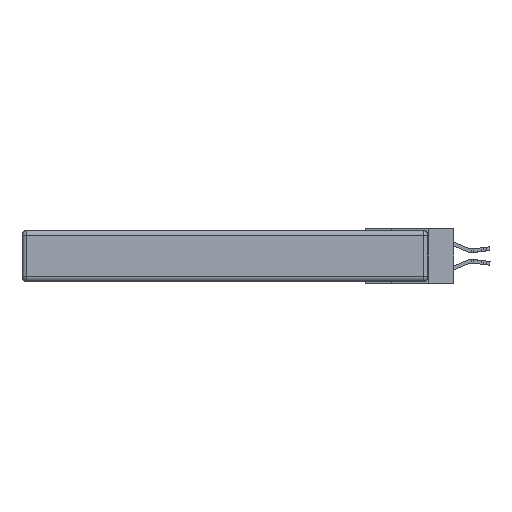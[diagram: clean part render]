
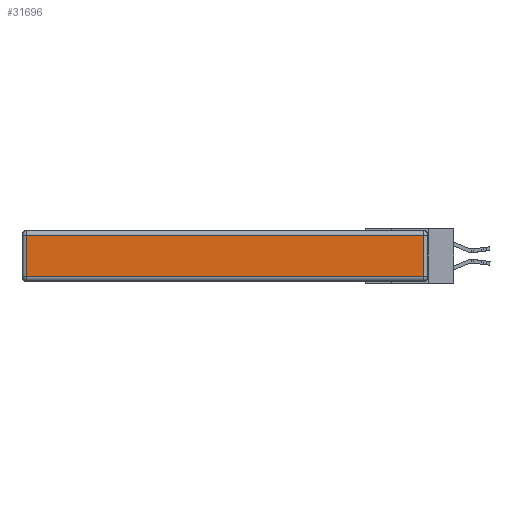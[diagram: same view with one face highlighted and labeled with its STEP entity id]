
A CAD part, left-side view. The second image highlights one B-rep face of the part: STEP entity #31696.
In plain terms, the highlighted planar face has unit normal (-1, 0, 0).
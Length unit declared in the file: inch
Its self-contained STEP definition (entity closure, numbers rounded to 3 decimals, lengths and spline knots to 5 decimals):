
#402 = DIRECTION ( 'NONE',  ( 0., 0., 1. ) ) ;
#422 = EDGE_LOOP ( 'NONE', ( #14379, #6504, #4582, #29925 ) ) ;
#1466 = CARTESIAN_POINT ( 'NONE',  ( 0., 0.03, -0.343 ) ) ;
#4254 = CARTESIAN_POINT ( 'NONE',  ( 0., 2.72, -0.03 ) ) ;
#4582 = ORIENTED_EDGE ( 'NONE', *, *, #23563, .T. ) ;
#4809 = DIRECTION ( 'NONE',  ( 0., 1., 0. ) ) ;
#5832 = PLANE ( 'NONE',  #35026 ) ;
#6318 = VERTEX_POINT ( 'NONE', #7643 ) ;
#6504 = ORIENTED_EDGE ( 'NONE', *, *, #9201, .T. ) ;
#7249 = DIRECTION ( 'NONE',  ( 0., -1., 0. ) ) ;
#7459 = VERTEX_POINT ( 'NONE', #20662 ) ;
#7643 = CARTESIAN_POINT ( 'NONE',  ( 0., 0.03, -0.313 ) ) ;
#9201 = EDGE_CURVE ( 'NONE', #6318, #14351, #9202, .T. ) ;
#9202 = LINE ( 'NONE', #1466, #26101 ) ;
#10902 = VECTOR ( 'NONE', #7249, 39.37008 ) ;
#13404 = CARTESIAN_POINT ( 'NONE',  ( 0., 0.03, -0.03 ) ) ;
#13429 = EDGE_CURVE ( 'NONE', #34975, #7459, #24948, .T. ) ;
#14351 = VERTEX_POINT ( 'NONE', #13404 ) ;
#14379 = ORIENTED_EDGE ( 'NONE', *, *, #17316, .T. ) ;
#17316 = EDGE_CURVE ( 'NONE', #7459, #6318, #21721, .T. ) ;
#19745 = VECTOR ( 'NONE', #34538, 39.37008 ) ;
#20662 = CARTESIAN_POINT ( 'NONE',  ( 0., 2.72, -0.313 ) ) ;
#21004 = CARTESIAN_POINT ( 'NONE',  ( 0., 0., -0.313 ) ) ;
#21721 = LINE ( 'NONE', #21004, #10902 ) ;
#23314 = VECTOR ( 'NONE', #4809, 39.37008 ) ;
#23563 = EDGE_CURVE ( 'NONE', #14351, #34975, #27179, .T. ) ;
#24202 = CARTESIAN_POINT ( 'NONE',  ( 0., 2.75, -0.03 ) ) ;
#24948 = LINE ( 'NONE', #34315, #19745 ) ;
#25180 = FACE_OUTER_BOUND ( 'NONE', #422, .T. ) ;
#26101 = VECTOR ( 'NONE', #26304, 39.37008 ) ;
#26304 = DIRECTION ( 'NONE',  ( 0., 0., 1. ) ) ;
#27179 = LINE ( 'NONE', #24202, #23314 ) ;
#28021 = CARTESIAN_POINT ( 'NONE',  ( 0., 0., -0.343 ) ) ;
#29925 = ORIENTED_EDGE ( 'NONE', *, *, #13429, .T. ) ;
#31696 = ADVANCED_FACE ( 'NONE', ( #25180 ), #5832, .T. ) ;
#33547 = DIRECTION ( 'NONE',  ( -1., 0., 0. ) ) ;
#34315 = CARTESIAN_POINT ( 'NONE',  ( 0., 2.72, -0.343 ) ) ;
#34538 = DIRECTION ( 'NONE',  ( 0., 0., -1. ) ) ;
#34975 = VERTEX_POINT ( 'NONE', #4254 ) ;
#35026 = AXIS2_PLACEMENT_3D ( 'NONE', #28021, #33547, #402 ) ;
